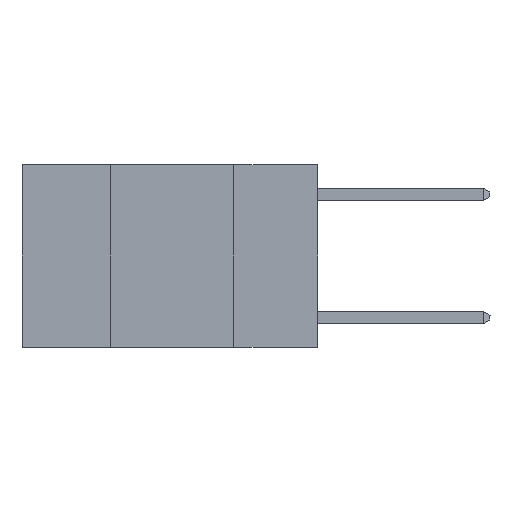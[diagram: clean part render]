
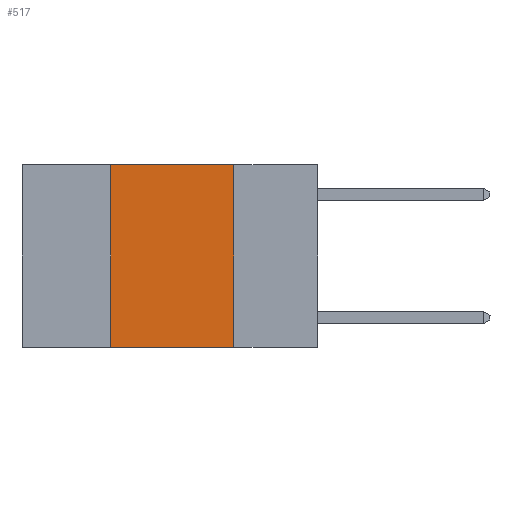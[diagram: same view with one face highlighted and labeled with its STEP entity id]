
A CAD part, left-side view. The second image highlights one B-rep face of the part: STEP entity #517.
In plain terms, the highlighted planar face has unit normal (-1, 0, 0).
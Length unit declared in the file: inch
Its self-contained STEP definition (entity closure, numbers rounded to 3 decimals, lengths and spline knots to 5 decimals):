
#55 = LINE ( 'NONE', #18893, #15650 ) ;
#517 = ADVANCED_FACE ( 'NONE', ( #23094 ), #11798, .F. ) ;
#906 = LINE ( 'NONE', #13970, #5080 ) ;
#2687 = DIRECTION ( 'NONE',  ( 0., -1., 0. ) ) ;
#3696 = CARTESIAN_POINT ( 'NONE',  ( 0., 0.6, 0. ) ) ;
#3732 = DIRECTION ( 'NONE',  ( 0., 0., 1. ) ) ;
#3998 = DIRECTION ( 'NONE',  ( 0., 0., -1. ) ) ;
#4969 = ORIENTED_EDGE ( 'NONE', *, *, #24847, .T. ) ;
#5080 = VECTOR ( 'NONE', #3732, 39.37008 ) ;
#5763 = DIRECTION ( 'NONE',  ( 0., 0., -1. ) ) ;
#6357 = EDGE_LOOP ( 'NONE', ( #16241, #23965, #18571, #4969 ) ) ;
#7173 = LINE ( 'NONE', #18185, #17297 ) ;
#7786 = EDGE_CURVE ( 'NONE', #16652, #25030, #906, .T. ) ;
#10397 = EDGE_CURVE ( 'NONE', #25030, #18576, #55, .T. ) ;
#11798 = PLANE ( 'NONE',  #22052 ) ;
#12945 = CARTESIAN_POINT ( 'NONE',  ( 0., 0.42, -0.37 ) ) ;
#13218 = LINE ( 'NONE', #15506, #18589 ) ;
#13970 = CARTESIAN_POINT ( 'NONE',  ( 0., 0.42, 0. ) ) ;
#14996 = EDGE_CURVE ( 'NONE', #18576, #23363, #7173, .T. ) ;
#15506 = CARTESIAN_POINT ( 'NONE',  ( 0., 0.6, -0.37 ) ) ;
#15650 = VECTOR ( 'NONE', #2687, 39.37008 ) ;
#16241 = ORIENTED_EDGE ( 'NONE', *, *, #14996, .F. ) ;
#16652 = VERTEX_POINT ( 'NONE', #12945 ) ;
#17297 = VECTOR ( 'NONE', #3998, 39.37008 ) ;
#17879 = DIRECTION ( 'NONE',  ( 1., 0., 0. ) ) ;
#18185 = CARTESIAN_POINT ( 'NONE',  ( 0., 0.17, 0. ) ) ;
#18571 = ORIENTED_EDGE ( 'NONE', *, *, #7786, .F. ) ;
#18576 = VERTEX_POINT ( 'NONE', #23036 ) ;
#18589 = VECTOR ( 'NONE', #25229, 39.37008 ) ;
#18893 = CARTESIAN_POINT ( 'NONE',  ( 0., 0.6, 0. ) ) ;
#21464 = CARTESIAN_POINT ( 'NONE',  ( 0., 0.17, -0.37 ) ) ;
#22052 = AXIS2_PLACEMENT_3D ( 'NONE', #3696, #17879, #5763 ) ;
#23036 = CARTESIAN_POINT ( 'NONE',  ( 0., 0.17, 0. ) ) ;
#23094 = FACE_OUTER_BOUND ( 'NONE', #6357, .T. ) ;
#23363 = VERTEX_POINT ( 'NONE', #21464 ) ;
#23885 = CARTESIAN_POINT ( 'NONE',  ( 0., 0.42, 0. ) ) ;
#23965 = ORIENTED_EDGE ( 'NONE', *, *, #10397, .F. ) ;
#24847 = EDGE_CURVE ( 'NONE', #16652, #23363, #13218, .T. ) ;
#25030 = VERTEX_POINT ( 'NONE', #23885 ) ;
#25229 = DIRECTION ( 'NONE',  ( 0., -1., 0. ) ) ;
